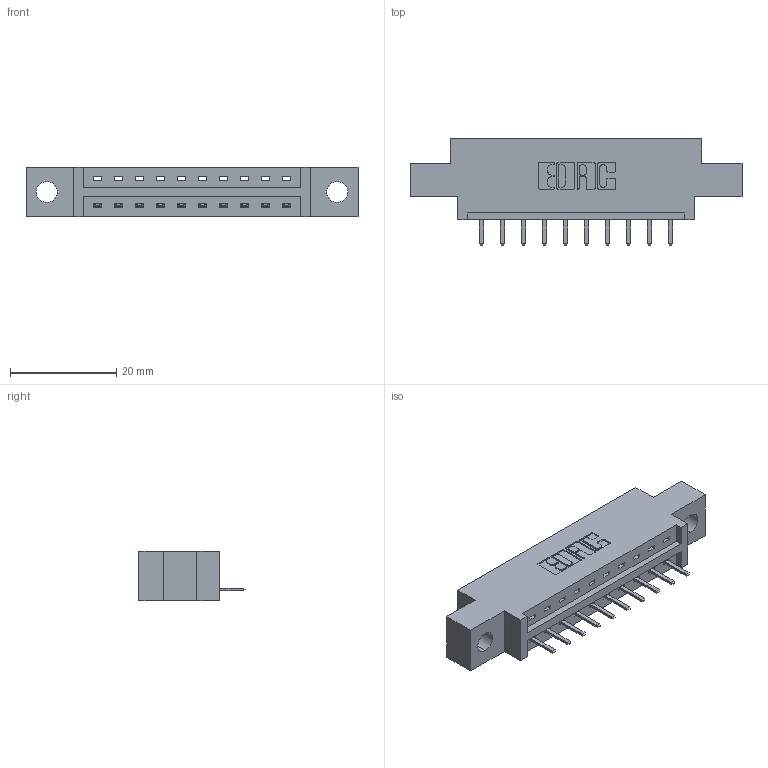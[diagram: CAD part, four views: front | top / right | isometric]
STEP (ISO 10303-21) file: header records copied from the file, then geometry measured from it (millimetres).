
FILE_DESCRIPTION (( 'STEP AP203' ), '1' );
FILE_NAME ('337-010-520-604.STEP', '2019-09-27T20:59:29', ( '' ), ( '' ), 'SwSTEP 2.0', 'SolidWorks 2016', '' );
FILE_SCHEMA (( 'CONFIG_CONTROL_DESIGN' ));
Length unit declared in the file: inch
Products named in the file (3): 345-292-001_345-293-120; 337 Part_0.170 Offset - 0.156 Dia-TH; 337-010-520-604
Assembly tree (11 placements, depth 2):
  337-010-520-604
    337 Part_0.170 Offset - 0.156 Dia-TH
    345-292-001_345-293-120  x10
Bounding box: 62.64 x 20.02 x 9.4 mm (x, y, z)
Volume: 5875.4 mm3; surface area: 5681.9 mm2
Topology: 11 solids, 11 shells, 778 faces, 2283 edges, 1494 vertices
Faces by surface type: plane 554, cylinder 224
Entity records: 11821 total; most frequent: CARTESIAN_POINT 2076, ORIENTED_EDGE 2010, DIRECTION 1801, EDGE_CURVE 1005, VECTOR 873, LINE 873, VERTEX_POINT 666, AXIS2_PLACEMENT_3D 464
